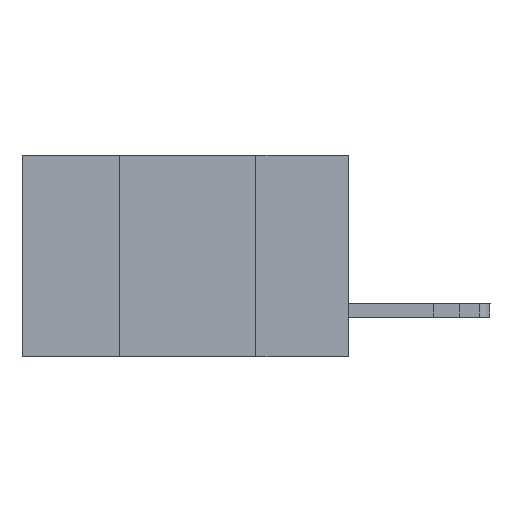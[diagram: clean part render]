
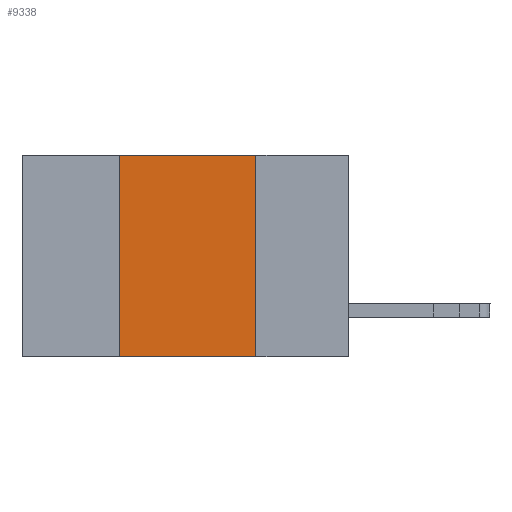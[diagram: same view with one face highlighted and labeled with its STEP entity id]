
A CAD part, left-side view. The second image highlights one B-rep face of the part: STEP entity #9338.
In plain terms, the highlighted planar face has unit normal (-1, 0, 0).
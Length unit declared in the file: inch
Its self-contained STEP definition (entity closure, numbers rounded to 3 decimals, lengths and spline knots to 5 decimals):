
#295 = VERTEX_POINT ( 'NONE', #8219 ) ;
#488 = VECTOR ( 'NONE', #8880, 39.37008 ) ;
#857 = EDGE_LOOP ( 'NONE', ( #2641, #10683, #4063, #7159 ) ) ;
#1190 = VERTEX_POINT ( 'NONE', #2995 ) ;
#1255 = LINE ( 'NONE', #5531, #488 ) ;
#1391 = EDGE_CURVE ( 'NONE', #295, #4793, #7636, .T. ) ;
#1699 = LINE ( 'NONE', #5098, #6384 ) ;
#1995 = CARTESIAN_POINT ( 'NONE',  ( 0., 0.17, 0. ) ) ;
#2596 = CARTESIAN_POINT ( 'NONE',  ( 0., 0.6, 0. ) ) ;
#2641 = ORIENTED_EDGE ( 'NONE', *, *, #2999, .F. ) ;
#2995 = CARTESIAN_POINT ( 'NONE',  ( 0., 0.42, -0.37 ) ) ;
#2999 = EDGE_CURVE ( 'NONE', #4793, #6004, #1699, .T. ) ;
#3404 = DIRECTION ( 'NONE',  ( 0., 0., -1. ) ) ;
#3779 = VECTOR ( 'NONE', #6598, 39.37008 ) ;
#3816 = AXIS2_PLACEMENT_3D ( 'NONE', #4293, #5278, #8625 ) ;
#4063 = ORIENTED_EDGE ( 'NONE', *, *, #8403, .F. ) ;
#4293 = CARTESIAN_POINT ( 'NONE',  ( 0., 0.6, 0. ) ) ;
#4793 = VERTEX_POINT ( 'NONE', #1995 ) ;
#5098 = CARTESIAN_POINT ( 'NONE',  ( 0., 0.17, -0.37 ) ) ;
#5212 = DIRECTION ( 'NONE',  ( 0., -1., 0. ) ) ;
#5278 = DIRECTION ( 'NONE',  ( 1., 0., 0. ) ) ;
#5434 = CARTESIAN_POINT ( 'NONE',  ( 0., 0.17, -0.37 ) ) ;
#5531 = CARTESIAN_POINT ( 'NONE',  ( 0., 0.42, -0.37 ) ) ;
#6004 = VERTEX_POINT ( 'NONE', #5434 ) ;
#6031 = CARTESIAN_POINT ( 'NONE',  ( 0., 0.6, -0.37 ) ) ;
#6384 = VECTOR ( 'NONE', #3404, 39.37008 ) ;
#6598 = DIRECTION ( 'NONE',  ( 0., -1., 0. ) ) ;
#7024 = PLANE ( 'NONE',  #3816 ) ;
#7159 = ORIENTED_EDGE ( 'NONE', *, *, #9782, .T. ) ;
#7636 = LINE ( 'NONE', #2596, #3779 ) ;
#8219 = CARTESIAN_POINT ( 'NONE',  ( 0., 0.42, 0. ) ) ;
#8403 = EDGE_CURVE ( 'NONE', #1190, #295, #1255, .T. ) ;
#8458 = FACE_OUTER_BOUND ( 'NONE', #857, .T. ) ;
#8553 = VECTOR ( 'NONE', #5212, 39.37008 ) ;
#8625 = DIRECTION ( 'NONE',  ( 0., 0., -1. ) ) ;
#8880 = DIRECTION ( 'NONE',  ( 0., 0., 1. ) ) ;
#9338 = ADVANCED_FACE ( 'NONE', ( #8458 ), #7024, .F. ) ;
#9473 = LINE ( 'NONE', #6031, #8553 ) ;
#9782 = EDGE_CURVE ( 'NONE', #1190, #6004, #9473, .T. ) ;
#10683 = ORIENTED_EDGE ( 'NONE', *, *, #1391, .F. ) ;
